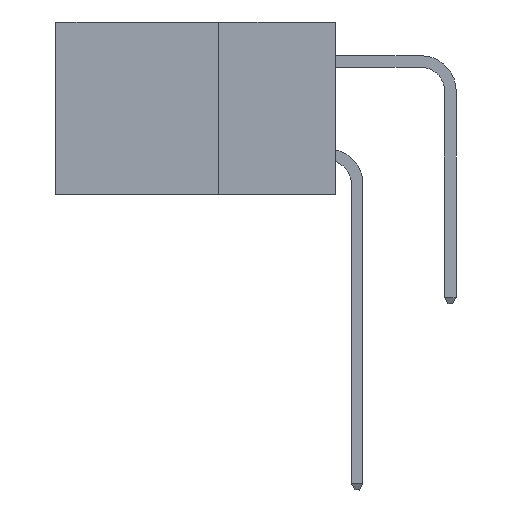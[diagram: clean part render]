
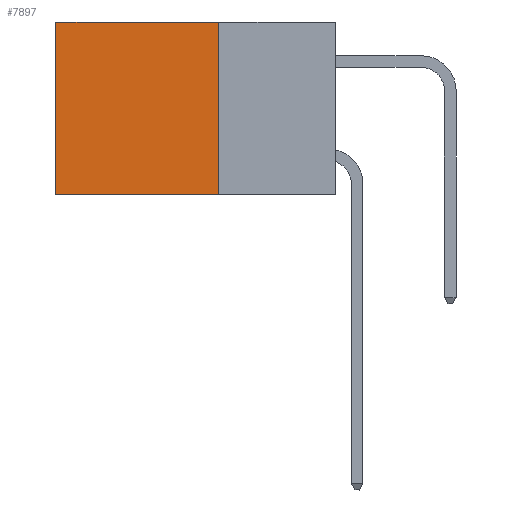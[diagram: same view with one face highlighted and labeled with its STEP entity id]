
A CAD part, left-side view. The second image highlights one B-rep face of the part: STEP entity #7897.
In plain terms, the highlighted planar face has unit normal (-1, 0, 0).
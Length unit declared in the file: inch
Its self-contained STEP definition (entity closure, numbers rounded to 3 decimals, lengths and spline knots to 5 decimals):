
#696 = DIRECTION ( 'NONE',  ( 0., 1., 0. ) ) ;
#1303 = VERTEX_POINT ( 'NONE', #7991 ) ;
#1347 = DIRECTION ( 'NONE',  ( 0., 0., -1. ) ) ;
#1814 = CARTESIAN_POINT ( 'NONE',  ( 0.2875, 0.6, 0. ) ) ;
#2290 = EDGE_CURVE ( 'NONE', #15505, #6543, #5704, .T. ) ;
#2357 = CARTESIAN_POINT ( 'NONE',  ( 0.2875, 0.25, 0. ) ) ;
#2652 = VECTOR ( 'NONE', #9160, 39.37008 ) ;
#2981 = ORIENTED_EDGE ( 'NONE', *, *, #6971, .T. ) ;
#3888 = FACE_OUTER_BOUND ( 'NONE', #9006, .T. ) ;
#4134 = LINE ( 'NONE', #14846, #2652 ) ;
#4479 = CARTESIAN_POINT ( 'NONE',  ( 0.2875, 0.25, 0. ) ) ;
#4602 = VECTOR ( 'NONE', #16075, 39.37008 ) ;
#4747 = CARTESIAN_POINT ( 'NONE',  ( 0.2875, 0.25, 0. ) ) ;
#5704 = LINE ( 'NONE', #4479, #8888 ) ;
#6543 = VERTEX_POINT ( 'NONE', #7541 ) ;
#6815 = ORIENTED_EDGE ( 'NONE', *, *, #15527, .T. ) ;
#6971 = EDGE_CURVE ( 'NONE', #15505, #10335, #7521, .T. ) ;
#7007 = CARTESIAN_POINT ( 'NONE',  ( 0.2875, 0.25, -0.37 ) ) ;
#7060 = ORIENTED_EDGE ( 'NONE', *, *, #8109, .F. ) ;
#7521 = LINE ( 'NONE', #4747, #4602 ) ;
#7541 = CARTESIAN_POINT ( 'NONE',  ( 0.2875, 0.25, -0.37 ) ) ;
#7897 = ADVANCED_FACE ( 'NONE', ( #3888 ), #15393, .F. ) ;
#7991 = CARTESIAN_POINT ( 'NONE',  ( 0.2875, 0.6, -0.37 ) ) ;
#8037 = VECTOR ( 'NONE', #696, 39.37008 ) ;
#8109 = EDGE_CURVE ( 'NONE', #6543, #1303, #13024, .T. ) ;
#8261 = DIRECTION ( 'NONE',  ( 0., 0., -1. ) ) ;
#8888 = VECTOR ( 'NONE', #8261, 39.37008 ) ;
#9006 = EDGE_LOOP ( 'NONE', ( #6815, #7060, #13302, #2981 ) ) ;
#9160 = DIRECTION ( 'NONE',  ( 0., 0., -1. ) ) ;
#10222 = CARTESIAN_POINT ( 'NONE',  ( 0.2875, 0.25, 0. ) ) ;
#10335 = VERTEX_POINT ( 'NONE', #1814 ) ;
#12942 = DIRECTION ( 'NONE',  ( 1., 0., 0. ) ) ;
#13024 = LINE ( 'NONE', #7007, #8037 ) ;
#13302 = ORIENTED_EDGE ( 'NONE', *, *, #2290, .F. ) ;
#14846 = CARTESIAN_POINT ( 'NONE',  ( 0.2875, 0.6, 0. ) ) ;
#15393 = PLANE ( 'NONE',  #16132 ) ;
#15505 = VERTEX_POINT ( 'NONE', #2357 ) ;
#15527 = EDGE_CURVE ( 'NONE', #10335, #1303, #4134, .T. ) ;
#16075 = DIRECTION ( 'NONE',  ( 0., 1., 0. ) ) ;
#16132 = AXIS2_PLACEMENT_3D ( 'NONE', #10222, #12942, #1347 ) ;
